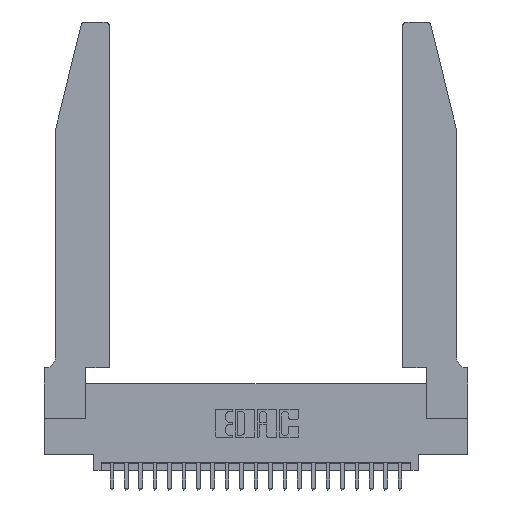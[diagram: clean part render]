
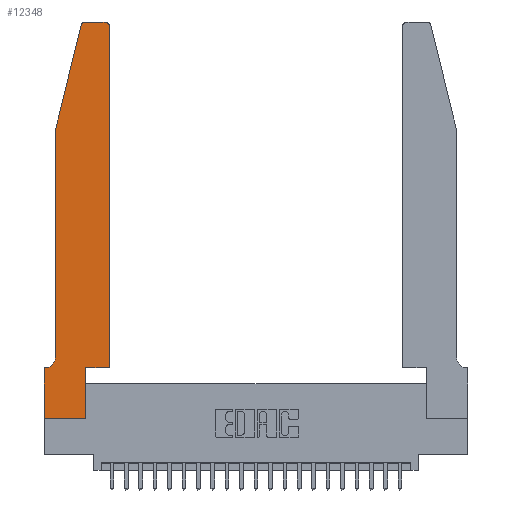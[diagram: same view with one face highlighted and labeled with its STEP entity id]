
A CAD part, top view. The second image highlights one B-rep face of the part: STEP entity #12348.
In plain terms, the highlighted planar face has unit normal (0, 0, 1).
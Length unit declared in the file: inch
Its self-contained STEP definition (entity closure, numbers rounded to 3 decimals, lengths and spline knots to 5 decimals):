
#165 = AXIS2_PLACEMENT_3D ( 'NONE', #23571, #16067, #21663 ) ;
#327 = CARTESIAN_POINT ( 'NONE',  ( 0.4505, 2.72, 0.37 ) ) ;
#350 = DIRECTION ( 'NONE',  ( -1., 0., 0. ) ) ;
#428 = CIRCLE ( 'NONE', #7071, 0.03 ) ;
#715 = CARTESIAN_POINT ( 'NONE',  ( 0., 0.35, 0.37 ) ) ;
#1469 = VERTEX_POINT ( 'NONE', #327 ) ;
#1828 = VERTEX_POINT ( 'NONE', #6879 ) ;
#1872 = CARTESIAN_POINT ( 'NONE',  ( 0.0755, 0.35, 0.37 ) ) ;
#2001 = DIRECTION ( 'NONE',  ( 0., 1., 0. ) ) ;
#2482 = EDGE_CURVE ( 'NONE', #11165, #7653, #2571, .T. ) ;
#2571 = LINE ( 'NONE', #11930, #5474 ) ;
#2750 = CARTESIAN_POINT ( 'NONE',  ( 0.0755, 2., 0.37 ) ) ;
#2955 = VECTOR ( 'NONE', #22326, 39.37008 ) ;
#3522 = CARTESIAN_POINT ( 'NONE',  ( 0.4205, 2.75, 0.37 ) ) ;
#3887 = VECTOR ( 'NONE', #5162, 39.37008 ) ;
#3894 = DIRECTION ( 'NONE',  ( 0., -1., 0. ) ) ;
#4203 = VERTEX_POINT ( 'NONE', #3522 ) ;
#4332 = LINE ( 'NONE', #1872, #6963 ) ;
#5162 = DIRECTION ( 'NONE',  ( -1., 0., 0. ) ) ;
#5474 = VECTOR ( 'NONE', #15690, 39.37008 ) ;
#5618 = CARTESIAN_POINT ( 'NONE',  ( 0.2865, 0.35, 0.37 ) ) ;
#6066 = FACE_OUTER_BOUND ( 'NONE', #18546, .T. ) ;
#6222 = LINE ( 'NONE', #22165, #3887 ) ;
#6405 = DIRECTION ( 'NONE',  ( 1., 0., 0. ) ) ;
#6825 = DIRECTION ( 'NONE',  ( 0., 0., 1. ) ) ;
#6879 = CARTESIAN_POINT ( 'NONE',  ( 0.25487, 2.72718, 0.37 ) ) ;
#6963 = VECTOR ( 'NONE', #350, 39.37008 ) ;
#7061 = ORIENTED_EDGE ( 'NONE', *, *, #22416, .T. ) ;
#7071 = AXIS2_PLACEMENT_3D ( 'NONE', #21604, #6825, #23510 ) ;
#7653 = VERTEX_POINT ( 'NONE', #11206 ) ;
#7999 = LINE ( 'NONE', #5618, #23216 ) ;
#8689 = CARTESIAN_POINT ( 'NONE',  ( 0.284, 2.75, 0.37 ) ) ;
#8958 = CARTESIAN_POINT ( 'NONE',  ( 0.0755, 2., 0.37 ) ) ;
#9327 = EDGE_CURVE ( 'NONE', #12773, #10691, #16503, .T. ) ;
#9508 = EDGE_CURVE ( 'NONE', #4203, #13017, #6222, .T. ) ;
#9984 = ORIENTED_EDGE ( 'NONE', *, *, #20989, .T. ) ;
#10036 = ORIENTED_EDGE ( 'NONE', *, *, #18579, .T. ) ;
#10316 = CARTESIAN_POINT ( 'NONE',  ( 0.2865, 0., 0.37 ) ) ;
#10691 = VERTEX_POINT ( 'NONE', #17171 ) ;
#10739 = ORIENTED_EDGE ( 'NONE', *, *, #13670, .T. ) ;
#10981 = AXIS2_PLACEMENT_3D ( 'NONE', #715, #13967, #6405 ) ;
#11064 = EDGE_CURVE ( 'NONE', #13095, #20246, #22219, .T. ) ;
#11165 = VERTEX_POINT ( 'NONE', #17091 ) ;
#11206 = CARTESIAN_POINT ( 'NONE',  ( 0., 0., 0.37 ) ) ;
#11468 = CARTESIAN_POINT ( 'NONE',  ( 0.4505, 0.35, 0.37 ) ) ;
#11816 = ORIENTED_EDGE ( 'NONE', *, *, #16689, .T. ) ;
#11930 = CARTESIAN_POINT ( 'NONE',  ( 0., 0., 0.37 ) ) ;
#12348 = ADVANCED_FACE ( 'NONE', ( #6066 ), #21444, .T. ) ;
#12611 = DIRECTION ( 'NONE',  ( 0., 0., -1. ) ) ;
#12773 = VERTEX_POINT ( 'NONE', #14655 ) ;
#12804 = ORIENTED_EDGE ( 'NONE', *, *, #9508, .T. ) ;
#13017 = VERTEX_POINT ( 'NONE', #8689 ) ;
#13095 = VERTEX_POINT ( 'NONE', #18606 ) ;
#13631 = DIRECTION ( 'NONE',  ( -0.239, -0.971, 0. ) ) ;
#13670 = EDGE_CURVE ( 'NONE', #1469, #4203, #428, .T. ) ;
#13967 = DIRECTION ( 'NONE',  ( 0., 0., 1. ) ) ;
#14566 = DIRECTION ( 'NONE',  ( -1., 0., 0. ) ) ;
#14587 = EDGE_CURVE ( 'NONE', #21442, #13095, #7999, .T. ) ;
#14655 = CARTESIAN_POINT ( 'NONE',  ( 0.0755, 0.42, 0.37 ) ) ;
#14964 = LINE ( 'NONE', #22520, #20739 ) ;
#15481 = EDGE_CURVE ( 'NONE', #1828, #16560, #22581, .T. ) ;
#15690 = DIRECTION ( 'NONE',  ( 0., -1., 0. ) ) ;
#16067 = DIRECTION ( 'NONE',  ( 0., 0., 1. ) ) ;
#16100 = CARTESIAN_POINT ( 'NONE',  ( 0.4505, 0.35, 0.37 ) ) ;
#16321 = ORIENTED_EDGE ( 'NONE', *, *, #9327, .T. ) ;
#16503 = CIRCLE ( 'NONE', #18152, 0.07 ) ;
#16560 = VERTEX_POINT ( 'NONE', #8958 ) ;
#16689 = EDGE_CURVE ( 'NONE', #7653, #21442, #21382, .T. ) ;
#17051 = VECTOR ( 'NONE', #13631, 39.37008 ) ;
#17091 = CARTESIAN_POINT ( 'NONE',  ( 0., 0.35, 0.37 ) ) ;
#17171 = CARTESIAN_POINT ( 'NONE',  ( 0.0055, 0.35, 0.37 ) ) ;
#17856 = EDGE_CURVE ( 'NONE', #10691, #11165, #4332, .T. ) ;
#18049 = VECTOR ( 'NONE', #2001, 39.37008 ) ;
#18152 = AXIS2_PLACEMENT_3D ( 'NONE', #20070, #12611, #14566 ) ;
#18546 = EDGE_LOOP ( 'NONE', ( #12804, #9984, #20668, #7061, #16321, #21752, #24074, #11816, #19263, #23171, #10036, #10739 ) ) ;
#18579 = EDGE_CURVE ( 'NONE', #20246, #1469, #22992, .T. ) ;
#18606 = CARTESIAN_POINT ( 'NONE',  ( 0.2865, 0.35, 0.37 ) ) ;
#18783 = DIRECTION ( 'NONE',  ( 0., 1., 0. ) ) ;
#18813 = CIRCLE ( 'NONE', #165, 0.03 ) ;
#19263 = ORIENTED_EDGE ( 'NONE', *, *, #14587, .T. ) ;
#20070 = CARTESIAN_POINT ( 'NONE',  ( 0.0055, 0.42, 0.37 ) ) ;
#20246 = VERTEX_POINT ( 'NONE', #16100 ) ;
#20581 = CARTESIAN_POINT ( 'NONE',  ( 0., 0., 0.37 ) ) ;
#20668 = ORIENTED_EDGE ( 'NONE', *, *, #15481, .T. ) ;
#20739 = VECTOR ( 'NONE', #3894, 39.37008 ) ;
#20989 = EDGE_CURVE ( 'NONE', #13017, #1828, #18813, .T. ) ;
#21382 = LINE ( 'NONE', #20581, #2955 ) ;
#21442 = VERTEX_POINT ( 'NONE', #10316 ) ;
#21444 = PLANE ( 'NONE',  #10981 ) ;
#21604 = CARTESIAN_POINT ( 'NONE',  ( 0.4205, 2.72, 0.37 ) ) ;
#21663 = DIRECTION ( 'NONE',  ( 1., 0., 0. ) ) ;
#21752 = ORIENTED_EDGE ( 'NONE', *, *, #17856, .T. ) ;
#22071 = DIRECTION ( 'NONE',  ( 1., 0., 0. ) ) ;
#22165 = CARTESIAN_POINT ( 'NONE',  ( 0.2605, 2.75, 0.37 ) ) ;
#22219 = LINE ( 'NONE', #23640, #23984 ) ;
#22326 = DIRECTION ( 'NONE',  ( 1., 0., 0. ) ) ;
#22416 = EDGE_CURVE ( 'NONE', #16560, #12773, #14964, .T. ) ;
#22520 = CARTESIAN_POINT ( 'NONE',  ( 0.0755, 2., 0.37 ) ) ;
#22581 = LINE ( 'NONE', #2750, #17051 ) ;
#22992 = LINE ( 'NONE', #11468, #18049 ) ;
#23171 = ORIENTED_EDGE ( 'NONE', *, *, #11064, .T. ) ;
#23216 = VECTOR ( 'NONE', #18783, 39.37008 ) ;
#23510 = DIRECTION ( 'NONE',  ( 1., 0., 0. ) ) ;
#23571 = CARTESIAN_POINT ( 'NONE',  ( 0.284, 2.72, 0.37 ) ) ;
#23640 = CARTESIAN_POINT ( 'NONE',  ( 0.4505, 0.35, 0.37 ) ) ;
#23984 = VECTOR ( 'NONE', #22071, 39.37008 ) ;
#24074 = ORIENTED_EDGE ( 'NONE', *, *, #2482, .T. ) ;
